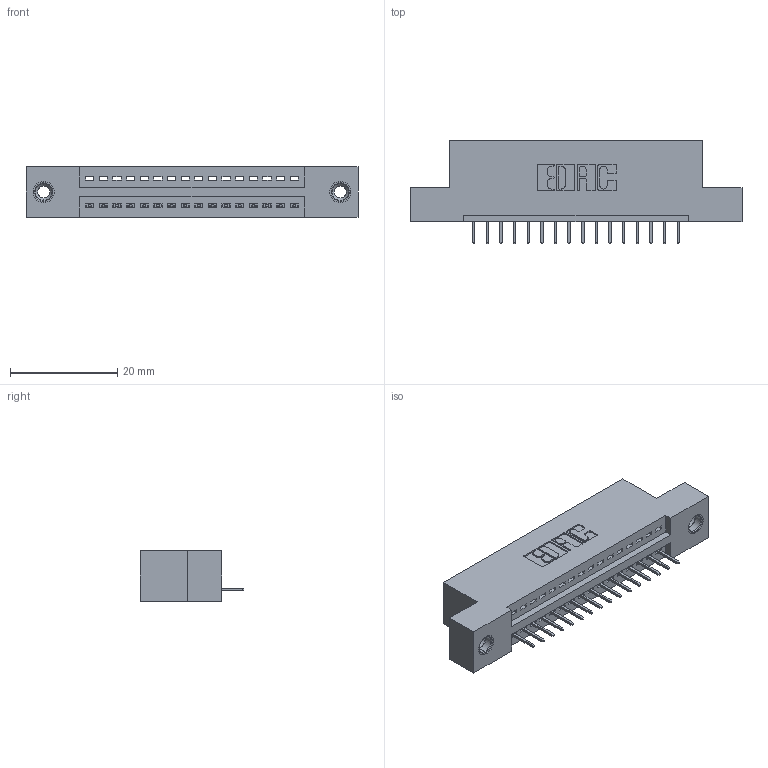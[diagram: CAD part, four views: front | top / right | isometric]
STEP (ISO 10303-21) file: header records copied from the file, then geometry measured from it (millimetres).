
FILE_DESCRIPTION (( 'STEP AP203' ), '1' );
FILE_NAME ('345-016-524-108.STEP', '2018-08-18T22:41:30', ( '' ), ( '' ), 'SwSTEP 2.0', 'SolidWorks 2016', '' );
FILE_SCHEMA (( 'CONFIG_CONTROL_DESIGN' ));
Length unit declared in the file: inch
Products named in the file (4): 345 Part_Flush Mounting Lugs - 0.156 Dia-TI; 345-292-001_345-293-124; 345-250-001_345-250-003-102; 345-016-524-108
Assembly tree (19 placements, depth 2):
  345-016-524-108
    345 Part_Flush Mounting Lugs - 0.156 Dia-TI
    345-292-001_345-293-124  x16
    345-250-001_345-250-003-102  x2
Bounding box: 61.85 x 19.35 x 9.4 mm (x, y, z)
Volume: 5591.8 mm3; surface area: 6894.7 mm2
Topology: 19 solids, 19 shells, 1178 faces, 3357 edges, 2166 vertices
Faces by surface type: plane 848, cylinder 314, cone 12, torus 4
Entity records: 16802 total; most frequent: CARTESIAN_POINT 2891, ORIENTED_EDGE 2834, DIRECTION 2591, EDGE_CURVE 1417, VECTOR 1205, LINE 1205, VERTEX_POINT 936, AXIS2_PLACEMENT_3D 693
